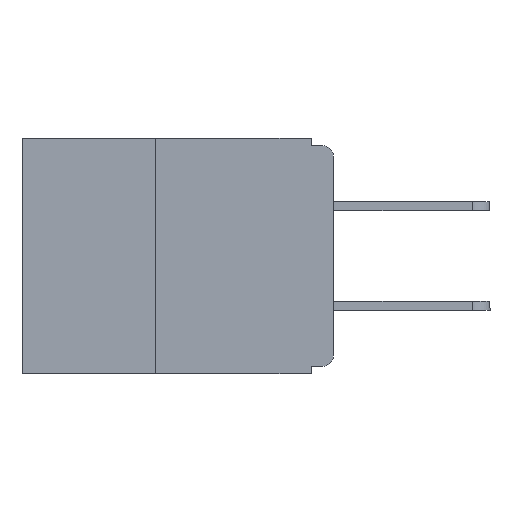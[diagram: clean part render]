
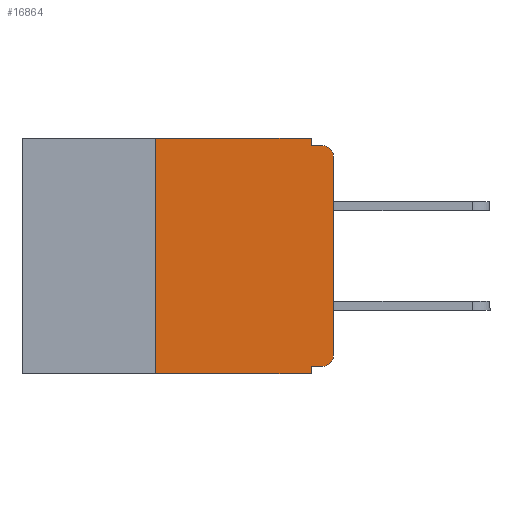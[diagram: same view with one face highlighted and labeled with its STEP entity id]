
A CAD part, left-side view. The second image highlights one B-rep face of the part: STEP entity #16864.
In plain terms, the highlighted planar face has unit normal (-1, 0, 0).
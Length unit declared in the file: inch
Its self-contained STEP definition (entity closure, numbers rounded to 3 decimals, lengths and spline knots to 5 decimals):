
#78 = LINE ( 'NONE', #5604, #20439 ) ;
#864 = CARTESIAN_POINT ( 'NONE',  ( 0., 0.25, -0.33 ) ) ;
#942 = DIRECTION ( 'NONE',  ( 0., 0., 1. ) ) ;
#1065 = CARTESIAN_POINT ( 'NONE',  ( 0., 0.437, 0. ) ) ;
#1164 = CARTESIAN_POINT ( 'NONE',  ( 0., 0., -0.01 ) ) ;
#1410 = VERTEX_POINT ( 'NONE', #15208 ) ;
#1848 = DIRECTION ( 'NONE',  ( 0., 0., -1. ) ) ;
#2026 = VERTEX_POINT ( 'NONE', #8334 ) ;
#2061 = LINE ( 'NONE', #11269, #14036 ) ;
#2279 = ORIENTED_EDGE ( 'NONE', *, *, #14134, .F. ) ;
#2310 = EDGE_CURVE ( 'NONE', #1410, #10368, #17914, .T. ) ;
#2456 = VERTEX_POINT ( 'NONE', #18744 ) ;
#2648 = LINE ( 'NONE', #1164, #7148 ) ;
#2847 = DIRECTION ( 'NONE',  ( 0., -1., 0. ) ) ;
#3585 = LINE ( 'NONE', #20002, #7549 ) ;
#3671 = DIRECTION ( 'NONE',  ( 0., 0., -1. ) ) ;
#3711 = DIRECTION ( 'NONE',  ( -1., 0., 0. ) ) ;
#3717 = CARTESIAN_POINT ( 'NONE',  ( 0., 0.015, -0.305 ) ) ;
#3728 = VERTEX_POINT ( 'NONE', #5163 ) ;
#3848 = EDGE_CURVE ( 'NONE', #15591, #6391, #15910, .T. ) ;
#3864 = ORIENTED_EDGE ( 'NONE', *, *, #16705, .T. ) ;
#4316 = EDGE_CURVE ( 'NONE', #2456, #8555, #3585, .T. ) ;
#4488 = ORIENTED_EDGE ( 'NONE', *, *, #3848, .T. ) ;
#4775 = DIRECTION ( 'NONE',  ( 0., 0., 1. ) ) ;
#4876 = CARTESIAN_POINT ( 'NONE',  ( 0., 0.25, 0. ) ) ;
#5163 = CARTESIAN_POINT ( 'NONE',  ( 0., 0.015, -0.01 ) ) ;
#5395 = ORIENTED_EDGE ( 'NONE', *, *, #5717, .T. ) ;
#5604 = CARTESIAN_POINT ( 'NONE',  ( 0., 0.031, 0. ) ) ;
#5717 = EDGE_CURVE ( 'NONE', #2026, #3728, #11061, .T. ) ;
#6013 = LINE ( 'NONE', #19176, #17600 ) ;
#6200 = CARTESIAN_POINT ( 'NONE',  ( 0., 0.031, 0. ) ) ;
#6391 = VERTEX_POINT ( 'NONE', #11846 ) ;
#6914 = VERTEX_POINT ( 'NONE', #6200 ) ;
#7148 = VECTOR ( 'NONE', #12725, 39.37008 ) ;
#7193 = CARTESIAN_POINT ( 'NONE',  ( 0., 0., -0.32 ) ) ;
#7316 = ORIENTED_EDGE ( 'NONE', *, *, #2310, .F. ) ;
#7459 = EDGE_LOOP ( 'NONE', ( #3864, #5395, #2279, #10386, #16871, #7316, #9759, #11880, #10736, #4488 ) ) ;
#7528 = EDGE_CURVE ( 'NONE', #15591, #2456, #15120, .T. ) ;
#7549 = VECTOR ( 'NONE', #19697, 39.37008 ) ;
#8334 = CARTESIAN_POINT ( 'NONE',  ( 0., 0., -0.025 ) ) ;
#8536 = CARTESIAN_POINT ( 'NONE',  ( 0., 0.437, 0. ) ) ;
#8555 = VERTEX_POINT ( 'NONE', #19134 ) ;
#9759 = ORIENTED_EDGE ( 'NONE', *, *, #10905, .T. ) ;
#10368 = VERTEX_POINT ( 'NONE', #4876 ) ;
#10386 = ORIENTED_EDGE ( 'NONE', *, *, #17007, .F. ) ;
#10736 = ORIENTED_EDGE ( 'NONE', *, *, #7528, .F. ) ;
#10905 = EDGE_CURVE ( 'NONE', #1410, #8555, #6013, .T. ) ;
#11061 = CIRCLE ( 'NONE', #19709, 0.015 ) ;
#11120 = FACE_OUTER_BOUND ( 'NONE', #7459, .T. ) ;
#11269 = CARTESIAN_POINT ( 'NONE',  ( 0., 0., 0. ) ) ;
#11750 = DIRECTION ( 'NONE',  ( 1., 0., 0. ) ) ;
#11846 = CARTESIAN_POINT ( 'NONE',  ( 0., 0., -0.305 ) ) ;
#11880 = ORIENTED_EDGE ( 'NONE', *, *, #4316, .F. ) ;
#12014 = DIRECTION ( 'NONE',  ( 0., 1., 0. ) ) ;
#12725 = DIRECTION ( 'NONE',  ( 0., -1., 0. ) ) ;
#12788 = LINE ( 'NONE', #1065, #20409 ) ;
#14036 = VECTOR ( 'NONE', #4775, 39.37008 ) ;
#14134 = EDGE_CURVE ( 'NONE', #15700, #3728, #2648, .T. ) ;
#14790 = PLANE ( 'NONE',  #16115 ) ;
#15120 = LINE ( 'NONE', #7193, #18690 ) ;
#15208 = CARTESIAN_POINT ( 'NONE',  ( 0., 0.25, -0.33 ) ) ;
#15591 = VERTEX_POINT ( 'NONE', #16154 ) ;
#15700 = VERTEX_POINT ( 'NONE', #17990 ) ;
#15910 = CIRCLE ( 'NONE', #17958, 0.015 ) ;
#16115 = AXIS2_PLACEMENT_3D ( 'NONE', #8536, #11750, #1848 ) ;
#16154 = CARTESIAN_POINT ( 'NONE',  ( 0., 0.015, -0.32 ) ) ;
#16586 = EDGE_CURVE ( 'NONE', #10368, #6914, #12788, .T. ) ;
#16705 = EDGE_CURVE ( 'NONE', #6391, #2026, #2061, .T. ) ;
#16864 = ADVANCED_FACE ( 'NONE', ( #11120 ), #14790, .F. ) ;
#16871 = ORIENTED_EDGE ( 'NONE', *, *, #16586, .F. ) ;
#17007 = EDGE_CURVE ( 'NONE', #6914, #15700, #78, .T. ) ;
#17600 = VECTOR ( 'NONE', #20676, 39.37008 ) ;
#17914 = LINE ( 'NONE', #864, #19292 ) ;
#17958 = AXIS2_PLACEMENT_3D ( 'NONE', #3717, #3711, #3671 ) ;
#17990 = CARTESIAN_POINT ( 'NONE',  ( 0., 0.031, -0.01 ) ) ;
#18140 = DIRECTION ( 'NONE',  ( 0., 0., -1. ) ) ;
#18143 = DIRECTION ( 'NONE',  ( -1., 0., 0. ) ) ;
#18162 = CARTESIAN_POINT ( 'NONE',  ( 0., 0.015, -0.025 ) ) ;
#18215 = DIRECTION ( 'NONE',  ( 0., 0., -1. ) ) ;
#18690 = VECTOR ( 'NONE', #12014, 39.37008 ) ;
#18744 = CARTESIAN_POINT ( 'NONE',  ( 0., 0.031, -0.32 ) ) ;
#19134 = CARTESIAN_POINT ( 'NONE',  ( 0., 0.031, -0.33 ) ) ;
#19176 = CARTESIAN_POINT ( 'NONE',  ( 0., 0.437, -0.33 ) ) ;
#19292 = VECTOR ( 'NONE', #942, 39.37008 ) ;
#19697 = DIRECTION ( 'NONE',  ( 0., 0., -1. ) ) ;
#19709 = AXIS2_PLACEMENT_3D ( 'NONE', #18162, #18143, #18140 ) ;
#20002 = CARTESIAN_POINT ( 'NONE',  ( 0., 0.031, -0.33 ) ) ;
#20409 = VECTOR ( 'NONE', #2847, 39.37008 ) ;
#20439 = VECTOR ( 'NONE', #18215, 39.37008 ) ;
#20676 = DIRECTION ( 'NONE',  ( 0., -1., 0. ) ) ;
